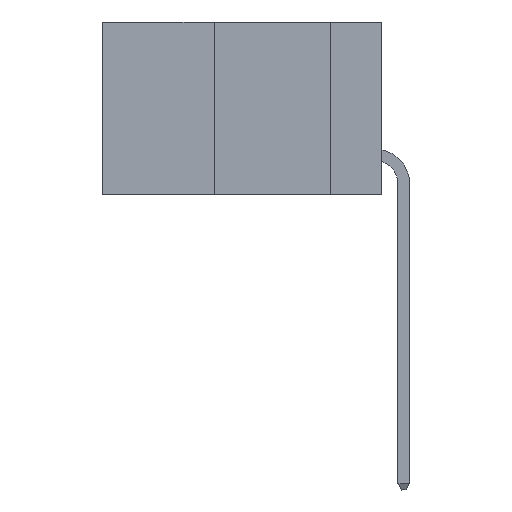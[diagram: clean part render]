
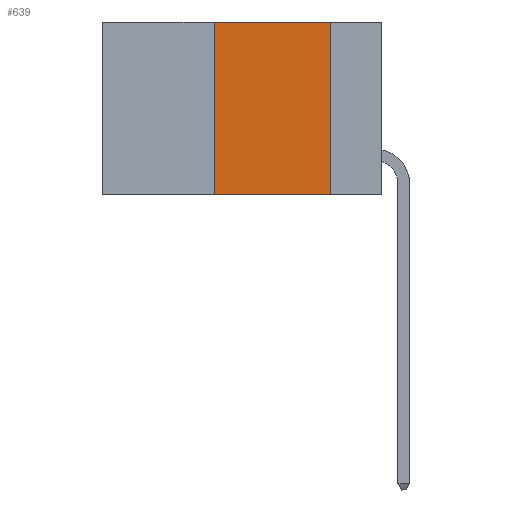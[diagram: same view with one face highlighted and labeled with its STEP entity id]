
A CAD part, left-side view. The second image highlights one B-rep face of the part: STEP entity #639.
In plain terms, the highlighted planar face has unit normal (-1, 0, 0).
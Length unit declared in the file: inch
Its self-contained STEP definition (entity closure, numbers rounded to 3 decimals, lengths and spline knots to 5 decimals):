
#639 = ADVANCED_FACE ( 'NONE', ( #7405 ), #18725, .F. ) ;
#1988 = EDGE_LOOP ( 'NONE', ( #3921, #13063, #12578, #19157 ) ) ;
#2319 = CARTESIAN_POINT ( 'NONE',  ( 0., 0.11, 0. ) ) ;
#2413 = DIRECTION ( 'NONE',  ( 0., 0., 1. ) ) ;
#2648 = LINE ( 'NONE', #15553, #11707 ) ;
#2750 = AXIS2_PLACEMENT_3D ( 'NONE', #15519, #5613, #12064 ) ;
#3147 = VERTEX_POINT ( 'NONE', #16306 ) ;
#3921 = ORIENTED_EDGE ( 'NONE', *, *, #11110, .F. ) ;
#4102 = VECTOR ( 'NONE', #11147, 39.37008 ) ;
#5364 = DIRECTION ( 'NONE',  ( 0., -1., 0. ) ) ;
#5613 = DIRECTION ( 'NONE',  ( 1., 0., 0. ) ) ;
#7405 = FACE_OUTER_BOUND ( 'NONE', #1988, .T. ) ;
#7764 = CARTESIAN_POINT ( 'NONE',  ( 0., 0.6, -0.37 ) ) ;
#8518 = LINE ( 'NONE', #7764, #4102 ) ;
#9134 = LINE ( 'NONE', #16700, #13544 ) ;
#10359 = EDGE_CURVE ( 'NONE', #12389, #14159, #9134, .T. ) ;
#11110 = EDGE_CURVE ( 'NONE', #14159, #12976, #2648, .T. ) ;
#11147 = DIRECTION ( 'NONE',  ( 0., -1., 0. ) ) ;
#11707 = VECTOR ( 'NONE', #18536, 39.37008 ) ;
#12019 = CARTESIAN_POINT ( 'NONE',  ( 0., 0.36, 0. ) ) ;
#12064 = DIRECTION ( 'NONE',  ( 0., 0., -1. ) ) ;
#12128 = EDGE_CURVE ( 'NONE', #3147, #12389, #13479, .T. ) ;
#12389 = VERTEX_POINT ( 'NONE', #12019 ) ;
#12578 = ORIENTED_EDGE ( 'NONE', *, *, #12128, .F. ) ;
#12681 = EDGE_CURVE ( 'NONE', #3147, #12976, #8518, .T. ) ;
#12942 = VECTOR ( 'NONE', #2413, 39.37008 ) ;
#12976 = VERTEX_POINT ( 'NONE', #18175 ) ;
#13063 = ORIENTED_EDGE ( 'NONE', *, *, #10359, .F. ) ;
#13479 = LINE ( 'NONE', #14504, #12942 ) ;
#13544 = VECTOR ( 'NONE', #5364, 39.37008 ) ;
#14159 = VERTEX_POINT ( 'NONE', #2319 ) ;
#14504 = CARTESIAN_POINT ( 'NONE',  ( 0., 0.36, 0. ) ) ;
#15519 = CARTESIAN_POINT ( 'NONE',  ( 0., 0.6, 0. ) ) ;
#15553 = CARTESIAN_POINT ( 'NONE',  ( 0., 0.11, 0. ) ) ;
#16306 = CARTESIAN_POINT ( 'NONE',  ( 0., 0.36, -0.37 ) ) ;
#16700 = CARTESIAN_POINT ( 'NONE',  ( 0., 0.6, 0. ) ) ;
#18175 = CARTESIAN_POINT ( 'NONE',  ( 0., 0.11, -0.37 ) ) ;
#18536 = DIRECTION ( 'NONE',  ( 0., 0., -1. ) ) ;
#18725 = PLANE ( 'NONE',  #2750 ) ;
#19157 = ORIENTED_EDGE ( 'NONE', *, *, #12681, .T. ) ;
